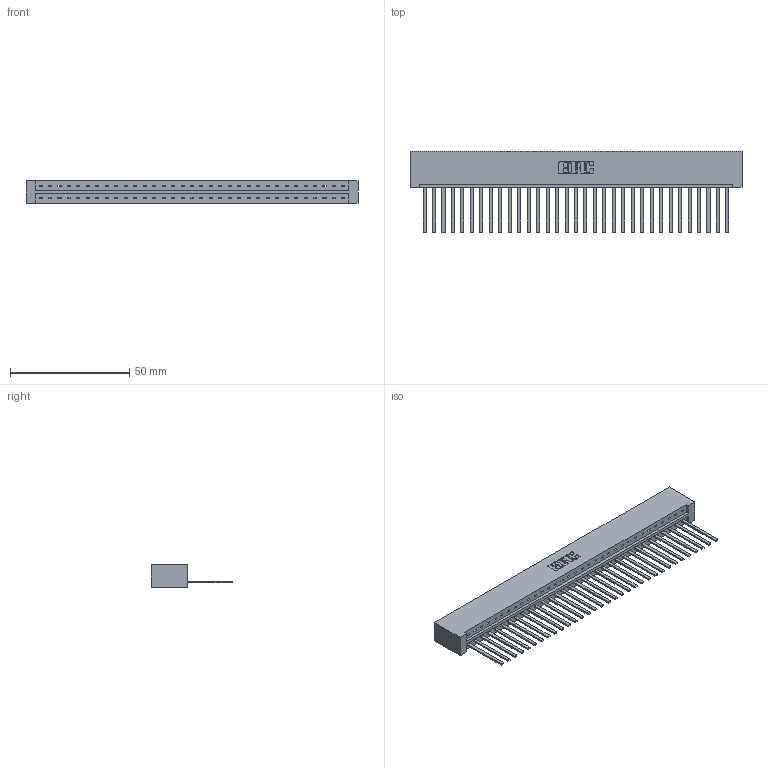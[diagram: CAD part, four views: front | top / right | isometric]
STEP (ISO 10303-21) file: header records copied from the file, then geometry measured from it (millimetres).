
FILE_DESCRIPTION (( 'STEP AP203' ), '1' );
FILE_NAME ('833-033-544-101.STEP', '2020-06-02T20:34:12', ( '' ), ( '' ), 'SwSTEP 2.0', 'SolidWorks 2020', '' );
FILE_SCHEMA (( 'CONFIG_CONTROL_DESIGN' ));
Length unit declared in the file: inch
Products named in the file (3): 345-292-001_345-293-144; 833 Part_Lugless; 833-033-544-101
Assembly tree (34 placements, depth 2):
  833-033-544-101
    833 Part_Lugless
    345-292-001_345-293-144  x33
Bounding box: 139.01 x 34.3 x 9.4 mm (x, y, z)
Volume: 14906.3 mm3; surface area: 17268.7 mm2
Topology: 34 solids, 34 shells, 1822 faces, 5501 edges, 3622 vertices
Faces by surface type: plane 1320, cylinder 502
Entity records: 20877 total; most frequent: CARTESIAN_POINT 3609, ORIENTED_EDGE 3578, DIRECTION 3051, EDGE_CURVE 1789, LINE 1673, VECTOR 1673, VERTEX_POINT 1190, AXIS2_PLACEMENT_3D 689
